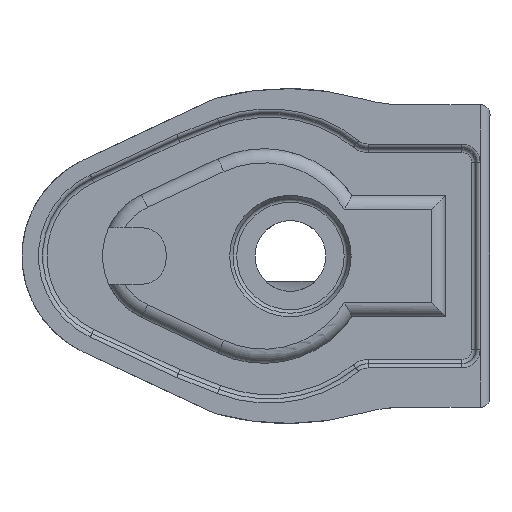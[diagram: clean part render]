
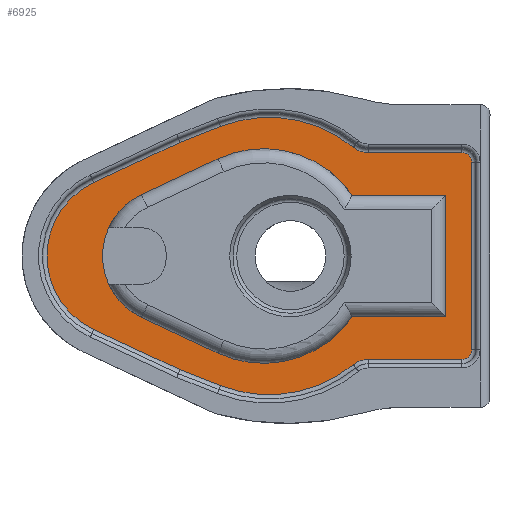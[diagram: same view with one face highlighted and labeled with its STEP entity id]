
A CAD part, left-side view. The second image highlights one B-rep face of the part: STEP entity #6925.
In plain terms, the highlighted planar face has unit normal (-1, 0, 0).
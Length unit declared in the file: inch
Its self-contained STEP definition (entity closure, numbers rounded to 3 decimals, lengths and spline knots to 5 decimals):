
#344=FACE_BOUND('',#990,.T.);
#360=PLANE('',#7429);
#537=FACE_OUTER_BOUND('',#989,.T.);
#989=EDGE_LOOP('',(#4586,#4587,#4588,#4589,#4590,#4591,#4592,#4593,#4594,
#4595,#4596,#4597,#4598,#4599));
#990=EDGE_LOOP('',(#4600,#4601,#4602,#4603,#4604,#4605,#4606,#4607));
#1518=CIRCLE('',#7384,0.94263);
#1521=CIRCLE('',#7388,0.1678);
#1525=CIRCLE('',#7394,0.07);
#1529=CIRCLE('',#7400,0.07);
#1533=CIRCLE('',#7406,0.1678);
#1536=CIRCLE('',#7410,0.94263);
#1539=CIRCLE('',#7415,0.57372);
#1545=CIRCLE('',#7430,0.76);
#1546=CIRCLE('',#7431,0.48);
#1547=CIRCLE('',#7432,0.76);
#1928=LINE('',#10310,#2332);
#1930=LINE('',#10319,#2334);
#1931=LINE('',#10337,#2335);
#1933=LINE('',#10349,#2337);
#1935=LINE('',#10361,#2339);
#1937=LINE('',#10376,#2341);
#1939=LINE('',#10385,#2343);
#1952=LINE('',#10420,#2356);
#1953=LINE('',#10422,#2357);
#1954=LINE('',#10424,#2358);
#1955=LINE('',#10428,#2359);
#1956=LINE('',#10432,#2360);
#2332=VECTOR('',#8223,0.3937);
#2334=VECTOR('',#8231,0.3937);
#2335=VECTOR('',#8254,0.3937);
#2337=VECTOR('',#8268,0.3937);
#2339=VECTOR('',#8282,0.3937);
#2341=VECTOR('',#8302,0.3937);
#2343=VECTOR('',#8314,0.3937);
#2356=VECTOR('',#8351,0.3937);
#2357=VECTOR('',#8352,0.3937);
#2358=VECTOR('',#8353,0.3937);
#2359=VECTOR('',#8356,0.3937);
#2360=VECTOR('',#8359,0.3937);
#2737=VERTEX_POINT('',#10307);
#2738=VERTEX_POINT('',#10309);
#2741=VERTEX_POINT('',#10316);
#2742=VERTEX_POINT('',#10318);
#2744=VERTEX_POINT('',#10323);
#2746=VERTEX_POINT('',#10329);
#2748=VERTEX_POINT('',#10335);
#2750=VERTEX_POINT('',#10341);
#2752=VERTEX_POINT('',#10347);
#2754=VERTEX_POINT('',#10353);
#2756=VERTEX_POINT('',#10359);
#2758=VERTEX_POINT('',#10365);
#2760=VERTEX_POINT('',#10371);
#2762=VERTEX_POINT('',#10380);
#2771=VERTEX_POINT('',#10418);
#2772=VERTEX_POINT('',#10419);
#2773=VERTEX_POINT('',#10421);
#2774=VERTEX_POINT('',#10423);
#2775=VERTEX_POINT('',#10425);
#2776=VERTEX_POINT('',#10427);
#2777=VERTEX_POINT('',#10429);
#2778=VERTEX_POINT('',#10431);
#3392=EDGE_CURVE('',#2737,#2738,#1928,.T.);
#3396=EDGE_CURVE('',#2741,#2742,#1930,.T.);
#3399=EDGE_CURVE('',#2744,#2741,#1518,.T.);
#3402=EDGE_CURVE('',#2746,#2744,#1521,.T.);
#3405=EDGE_CURVE('',#2748,#2746,#1931,.T.);
#3408=EDGE_CURVE('',#2750,#2748,#1525,.T.);
#3411=EDGE_CURVE('',#2752,#2750,#1933,.T.);
#3414=EDGE_CURVE('',#2754,#2752,#1529,.T.);
#3417=EDGE_CURVE('',#2756,#2754,#1935,.T.);
#3420=EDGE_CURVE('',#2758,#2756,#1533,.T.);
#3423=EDGE_CURVE('',#2760,#2758,#1536,.T.);
#3425=EDGE_CURVE('',#2738,#2760,#1937,.T.);
#3428=EDGE_CURVE('',#2762,#2737,#1539,.T.);
#3430=EDGE_CURVE('',#2742,#2762,#1939,.T.);
#3447=EDGE_CURVE('',#2771,#2772,#1952,.T.);
#3448=EDGE_CURVE('',#2773,#2772,#1953,.T.);
#3449=EDGE_CURVE('',#2773,#2774,#1954,.T.);
#3450=EDGE_CURVE('',#2774,#2775,#1545,.T.);
#3451=EDGE_CURVE('',#2775,#2776,#1955,.T.);
#3452=EDGE_CURVE('',#2776,#2777,#1546,.T.);
#3453=EDGE_CURVE('',#2777,#2778,#1956,.T.);
#3454=EDGE_CURVE('',#2778,#2771,#1547,.T.);
#4586=ORIENTED_EDGE('',*,*,#3396,.F.);
#4587=ORIENTED_EDGE('',*,*,#3399,.F.);
#4588=ORIENTED_EDGE('',*,*,#3402,.F.);
#4589=ORIENTED_EDGE('',*,*,#3405,.F.);
#4590=ORIENTED_EDGE('',*,*,#3408,.F.);
#4591=ORIENTED_EDGE('',*,*,#3411,.F.);
#4592=ORIENTED_EDGE('',*,*,#3414,.F.);
#4593=ORIENTED_EDGE('',*,*,#3417,.F.);
#4594=ORIENTED_EDGE('',*,*,#3420,.F.);
#4595=ORIENTED_EDGE('',*,*,#3423,.F.);
#4596=ORIENTED_EDGE('',*,*,#3425,.F.);
#4597=ORIENTED_EDGE('',*,*,#3392,.F.);
#4598=ORIENTED_EDGE('',*,*,#3428,.F.);
#4599=ORIENTED_EDGE('',*,*,#3430,.F.);
#4600=ORIENTED_EDGE('',*,*,#3447,.T.);
#4601=ORIENTED_EDGE('',*,*,#3448,.F.);
#4602=ORIENTED_EDGE('',*,*,#3449,.T.);
#4603=ORIENTED_EDGE('',*,*,#3450,.T.);
#4604=ORIENTED_EDGE('',*,*,#3451,.T.);
#4605=ORIENTED_EDGE('',*,*,#3452,.T.);
#4606=ORIENTED_EDGE('',*,*,#3453,.T.);
#4607=ORIENTED_EDGE('',*,*,#3454,.T.);
#6925=ADVANCED_FACE('',(#537,#344),#360,.F.);
#7384=AXIS2_PLACEMENT_3D('',#10325,#8238,#8239);
#7388=AXIS2_PLACEMENT_3D('',#10331,#8246,#8247);
#7394=AXIS2_PLACEMENT_3D('',#10343,#8260,#8261);
#7400=AXIS2_PLACEMENT_3D('',#10355,#8274,#8275);
#7406=AXIS2_PLACEMENT_3D('',#10367,#8288,#8289);
#7410=AXIS2_PLACEMENT_3D('',#10373,#8296,#8297);
#7415=AXIS2_PLACEMENT_3D('',#10382,#8308,#8309);
#7429=AXIS2_PLACEMENT_3D('',#10417,#8349,#8350);
#7430=AXIS2_PLACEMENT_3D('',#10426,#8354,#8355);
#7431=AXIS2_PLACEMENT_3D('',#10430,#8357,#8358);
#7432=AXIS2_PLACEMENT_3D('',#10433,#8360,#8361);
#8223=DIRECTION('',(0.,-0.906,0.423));
#8231=DIRECTION('',(0.,0.931,0.364));
#8238=DIRECTION('center_axis',(1.,0.,0.));
#8239=DIRECTION('ref_axis',(0.,-0.155,-0.988));
#8246=DIRECTION('center_axis',(-1.,0.,0.));
#8247=DIRECTION('ref_axis',(0.,0.335,0.942));
#8254=DIRECTION('',(0.,1.,0.));
#8260=DIRECTION('center_axis',(1.,0.,0.));
#8261=DIRECTION('ref_axis',(0.,-0.707,-0.707));
#8268=DIRECTION('',(0.,0.,-1.));
#8274=DIRECTION('center_axis',(1.,0.,0.));
#8275=DIRECTION('ref_axis',(0.,-0.707,0.707));
#8282=DIRECTION('',(0.,-1.,0.));
#8288=DIRECTION('center_axis',(-1.,0.,0.));
#8289=DIRECTION('ref_axis',(0.,0.335,-0.942));
#8296=DIRECTION('center_axis',(1.,0.,0.));
#8297=DIRECTION('ref_axis',(0.,-0.155,0.988));
#8302=DIRECTION('',(0.,-0.931,0.364));
#8308=DIRECTION('center_axis',(1.,0.,0.));
#8309=DIRECTION('ref_axis',(0.,1.,0.));
#8314=DIRECTION('',(0.,0.906,0.423));
#8349=DIRECTION('center_axis',(1.,0.,0.));
#8350=DIRECTION('ref_axis',(0.,0.,-1.));
#8351=DIRECTION('',(0.,-1.,0.));
#8352=DIRECTION('',(0.,0.,1.));
#8353=DIRECTION('',(0.,1.,0.));
#8354=DIRECTION('center_axis',(1.,0.,0.));
#8355=DIRECTION('ref_axis',(0.,0.,1.));
#8356=DIRECTION('',(0.,0.906,0.424));
#8357=DIRECTION('center_axis',(1.,0.,0.));
#8358=DIRECTION('ref_axis',(0.,0.,1.));
#8359=DIRECTION('',(0.,-0.906,0.424));
#8360=DIRECTION('center_axis',(1.,0.,0.));
#8361=DIRECTION('ref_axis',(0.,0.,1.));
#10307=CARTESIAN_POINT('',(0.,1.29247,0.51997));
#10309=CARTESIAN_POINT('',(0.,0.68094,0.80513));
#10310=CARTESIAN_POINT('',(0.,1.0789,0.61956));
#10316=CARTESIAN_POINT('',(0.,0.39439,-0.91722));
#10318=CARTESIAN_POINT('',(0.,0.68094,-0.80513));
#10319=CARTESIAN_POINT('',(0.,0.75251,-0.77713));
#10323=CARTESIAN_POINT('',(0.,-0.54423,-0.77031));
#10325=CARTESIAN_POINT('Origin',(0.,0.05099,-0.03937));
#10329=CARTESIAN_POINT('',(0.,-0.65018,-0.73263));
#10331=CARTESIAN_POINT('Origin',(0.,-0.65018,-0.90043));
#10335=CARTESIAN_POINT('',(0.,-1.31299,-0.73263));
#10337=CARTESIAN_POINT('',(0.,-0.06009,-0.73263));
#10341=CARTESIAN_POINT('',(0.,-1.38299,-0.66263));
#10343=CARTESIAN_POINT('Origin',(0.,-1.31299,-0.66263));
#10347=CARTESIAN_POINT('',(0.,-1.38299,0.66263));
#10349=CARTESIAN_POINT('',(0.,-1.38299,0.));
#10353=CARTESIAN_POINT('',(0.,-1.31299,0.73263));
#10355=CARTESIAN_POINT('Origin',(0.,-1.31299,0.66263));
#10359=CARTESIAN_POINT('',(0.,-0.65018,0.73263));
#10361=CARTESIAN_POINT('',(0.,-0.06009,0.73263));
#10365=CARTESIAN_POINT('',(0.,-0.54423,0.77031));
#10367=CARTESIAN_POINT('Origin',(0.,-0.65018,0.90043));
#10371=CARTESIAN_POINT('',(0.,0.39439,0.91722));
#10373=CARTESIAN_POINT('Origin',(0.,0.05099,0.03937));
#10376=CARTESIAN_POINT('',(0.,0.75251,0.77713));
#10380=CARTESIAN_POINT('',(0.,1.29247,-0.51997));
#10382=CARTESIAN_POINT('Origin',(0.,1.05,0.));
#10385=CARTESIAN_POINT('',(0.,0.76136,-0.76763));
#10417=CARTESIAN_POINT('Origin',(0.,0.53,0.));
#10418=CARTESIAN_POINT('',(0.,-0.53666,0.43));
#10419=CARTESIAN_POINT('',(0.,-1.2,0.43));
#10420=CARTESIAN_POINT('',(0.,-0.53666,0.43));
#10421=CARTESIAN_POINT('',(0.,-1.2,-0.43));
#10422=CARTESIAN_POINT('',(0.,-1.2,0.));
#10423=CARTESIAN_POINT('',(0.,-0.53666,-0.43));
#10424=CARTESIAN_POINT('',(0.,-1.2,-0.43));
#10425=CARTESIAN_POINT('',(0.,0.41242,-0.68822));
#10426=CARTESIAN_POINT('Origin',(0.,0.09,0.));
#10427=CARTESIAN_POINT('',(0.,0.95364,-0.43466));
#10428=CARTESIAN_POINT('',(0.,0.86343,-0.47692));
#10429=CARTESIAN_POINT('',(0.,0.95364,0.43466));
#10430=CARTESIAN_POINT('Origin',(0.,0.75,0.));
#10431=CARTESIAN_POINT('',(0.,0.41242,0.68822));
#10432=CARTESIAN_POINT('',(0.,0.59283,0.6037));
#10433=CARTESIAN_POINT('Origin',(0.,0.09,0.));
